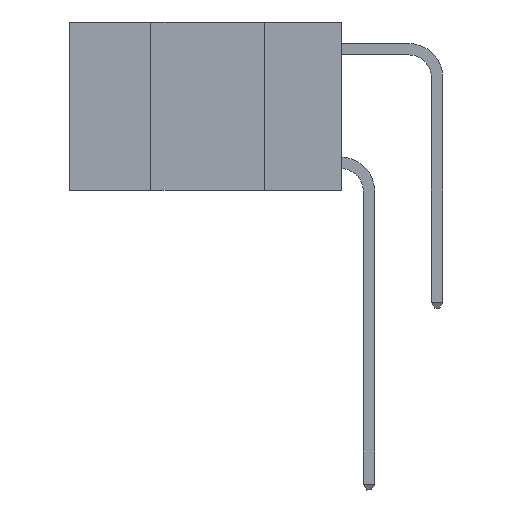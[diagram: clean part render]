
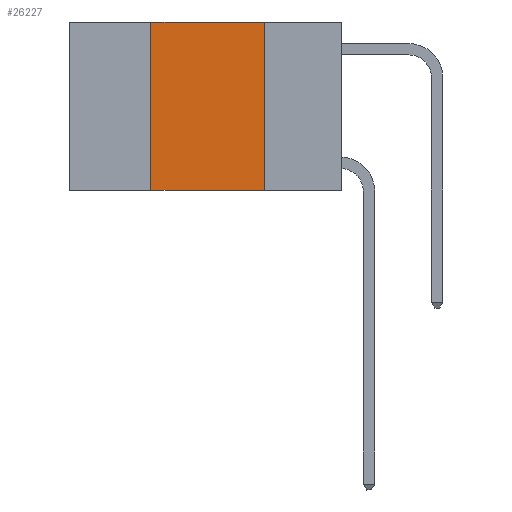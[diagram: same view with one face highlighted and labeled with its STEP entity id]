
A CAD part, left-side view. The second image highlights one B-rep face of the part: STEP entity #26227.
In plain terms, the highlighted planar face has unit normal (-1, 0, 0).
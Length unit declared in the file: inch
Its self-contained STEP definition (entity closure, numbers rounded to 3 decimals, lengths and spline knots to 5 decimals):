
#503 = DIRECTION ( 'NONE',  ( 0., 0., -1. ) ) ;
#560 = ORIENTED_EDGE ( 'NONE', *, *, #3617, .F. ) ;
#1421 = DIRECTION ( 'NONE',  ( 0., 0., 1. ) ) ;
#1460 = EDGE_CURVE ( 'NONE', #20510, #24913, #24631, .T. ) ;
#1786 = LINE ( 'NONE', #14068, #12751 ) ;
#3127 = CARTESIAN_POINT ( 'NONE',  ( 0., 0.6, 0. ) ) ;
#3270 = DIRECTION ( 'NONE',  ( 0., 0., -1. ) ) ;
#3617 = EDGE_CURVE ( 'NONE', #12284, #8714, #26835, .T. ) ;
#5596 = VECTOR ( 'NONE', #9716, 39.37008 ) ;
#7401 = ORIENTED_EDGE ( 'NONE', *, *, #1460, .F. ) ;
#8714 = VERTEX_POINT ( 'NONE', #21596 ) ;
#9144 = ORIENTED_EDGE ( 'NONE', *, *, #24667, .T. ) ;
#9716 = DIRECTION ( 'NONE',  ( 0., -1., 0. ) ) ;
#10850 = ORIENTED_EDGE ( 'NONE', *, *, #12383, .F. ) ;
#10975 = CARTESIAN_POINT ( 'NONE',  ( 0., 0.17, 0. ) ) ;
#11850 = DIRECTION ( 'NONE',  ( 0., -1., 0. ) ) ;
#11964 = AXIS2_PLACEMENT_3D ( 'NONE', #20202, #13650, #503 ) ;
#12284 = VERTEX_POINT ( 'NONE', #24746 ) ;
#12383 = EDGE_CURVE ( 'NONE', #8714, #20510, #17319, .T. ) ;
#12751 = VECTOR ( 'NONE', #11850, 39.37008 ) ;
#12910 = VECTOR ( 'NONE', #3270, 39.37008 ) ;
#13650 = DIRECTION ( 'NONE',  ( 1., 0., 0. ) ) ;
#14068 = CARTESIAN_POINT ( 'NONE',  ( 0., 0.6, -0.37 ) ) ;
#15788 = PLANE ( 'NONE',  #11964 ) ;
#17319 = LINE ( 'NONE', #3127, #5596 ) ;
#18654 = CARTESIAN_POINT ( 'NONE',  ( 0., 0.17, 0. ) ) ;
#18875 = EDGE_LOOP ( 'NONE', ( #7401, #10850, #560, #9144 ) ) ;
#19274 = CARTESIAN_POINT ( 'NONE',  ( 0., 0.17, -0.37 ) ) ;
#20202 = CARTESIAN_POINT ( 'NONE',  ( 0., 0.6, 0. ) ) ;
#20249 = FACE_OUTER_BOUND ( 'NONE', #18875, .T. ) ;
#20510 = VERTEX_POINT ( 'NONE', #10975 ) ;
#20972 = VECTOR ( 'NONE', #1421, 39.37008 ) ;
#21108 = CARTESIAN_POINT ( 'NONE',  ( 0., 0.42, 0. ) ) ;
#21596 = CARTESIAN_POINT ( 'NONE',  ( 0., 0.42, 0. ) ) ;
#24631 = LINE ( 'NONE', #18654, #12910 ) ;
#24667 = EDGE_CURVE ( 'NONE', #12284, #24913, #1786, .T. ) ;
#24746 = CARTESIAN_POINT ( 'NONE',  ( 0., 0.42, -0.37 ) ) ;
#24913 = VERTEX_POINT ( 'NONE', #19274 ) ;
#26227 = ADVANCED_FACE ( 'NONE', ( #20249 ), #15788, .F. ) ;
#26835 = LINE ( 'NONE', #21108, #20972 ) ;
